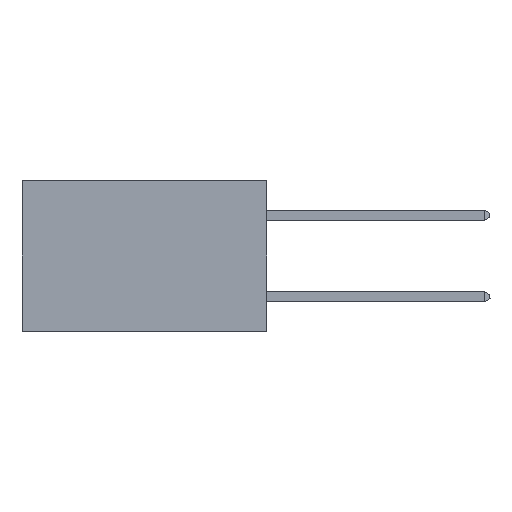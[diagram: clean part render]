
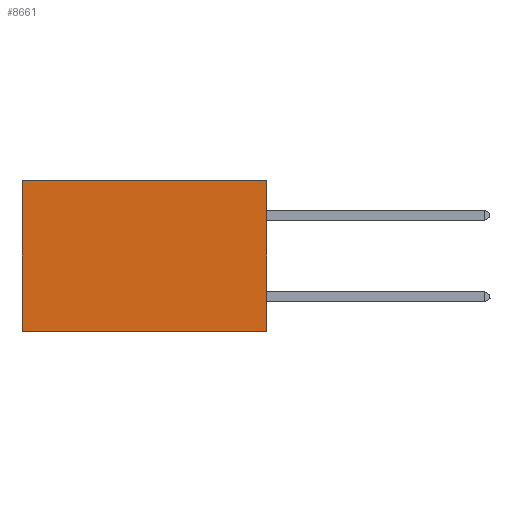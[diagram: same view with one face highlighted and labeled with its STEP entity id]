
A CAD part, left-side view. The second image highlights one B-rep face of the part: STEP entity #8661.
In plain terms, the highlighted planar face has unit normal (-1, 0, 0).
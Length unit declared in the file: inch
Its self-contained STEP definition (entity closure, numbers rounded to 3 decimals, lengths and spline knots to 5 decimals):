
#199 = CARTESIAN_POINT ( 'NONE',  ( 0.2875, 0., 0. ) ) ;
#417 = DIRECTION ( 'NONE',  ( 0., 0., -1. ) ) ;
#647 = VERTEX_POINT ( 'NONE', #5409 ) ;
#757 = EDGE_CURVE ( 'NONE', #14432, #23924, #18991, .T. ) ;
#1825 = LINE ( 'NONE', #18418, #25179 ) ;
#2025 = EDGE_CURVE ( 'NONE', #14432, #647, #1825, .T. ) ;
#2281 = VECTOR ( 'NONE', #417, 39.37008 ) ;
#3078 = VECTOR ( 'NONE', #3971, 39.37008 ) ;
#3748 = DIRECTION ( 'NONE',  ( 0., 0., -1. ) ) ;
#3971 = DIRECTION ( 'NONE',  ( 0., 1., 0. ) ) ;
#5409 = CARTESIAN_POINT ( 'NONE',  ( 0.2875, 0.6, 0. ) ) ;
#6171 = ORIENTED_EDGE ( 'NONE', *, *, #2025, .T. ) ;
#7472 = LINE ( 'NONE', #12927, #16571 ) ;
#7997 = FACE_OUTER_BOUND ( 'NONE', #15832, .T. ) ;
#8407 = PLANE ( 'NONE',  #21368 ) ;
#8661 = ADVANCED_FACE ( 'NONE', ( #7997 ), #8407, .F. ) ;
#9837 = EDGE_CURVE ( 'NONE', #23924, #15909, #25372, .T. ) ;
#9933 = ORIENTED_EDGE ( 'NONE', *, *, #757, .F. ) ;
#10668 = CARTESIAN_POINT ( 'NONE',  ( 0.2875, 0., 0. ) ) ;
#11431 = CARTESIAN_POINT ( 'NONE',  ( 0.2875, 0., 0. ) ) ;
#12497 = ORIENTED_EDGE ( 'NONE', *, *, #9837, .F. ) ;
#12574 = CARTESIAN_POINT ( 'NONE',  ( 0.2875, 0., -0.37 ) ) ;
#12927 = CARTESIAN_POINT ( 'NONE',  ( 0.2875, 0.6, 0. ) ) ;
#14432 = VERTEX_POINT ( 'NONE', #199 ) ;
#14695 = CARTESIAN_POINT ( 'NONE',  ( 0.2875, 0.6, -0.37 ) ) ;
#15832 = EDGE_LOOP ( 'NONE', ( #23559, #12497, #9933, #6171 ) ) ;
#15909 = VERTEX_POINT ( 'NONE', #14695 ) ;
#16571 = VECTOR ( 'NONE', #28467, 39.37008 ) ;
#16715 = EDGE_CURVE ( 'NONE', #647, #15909, #7472, .T. ) ;
#18418 = CARTESIAN_POINT ( 'NONE',  ( 0.2875, 0., 0. ) ) ;
#18991 = LINE ( 'NONE', #11431, #2281 ) ;
#21298 = CARTESIAN_POINT ( 'NONE',  ( 0.2875, 0., -0.37 ) ) ;
#21368 = AXIS2_PLACEMENT_3D ( 'NONE', #10668, #28075, #3748 ) ;
#23559 = ORIENTED_EDGE ( 'NONE', *, *, #16715, .T. ) ;
#23924 = VERTEX_POINT ( 'NONE', #21298 ) ;
#25118 = DIRECTION ( 'NONE',  ( 0., 1., 0. ) ) ;
#25179 = VECTOR ( 'NONE', #25118, 39.37008 ) ;
#25372 = LINE ( 'NONE', #12574, #3078 ) ;
#28075 = DIRECTION ( 'NONE',  ( 1., 0., 0. ) ) ;
#28467 = DIRECTION ( 'NONE',  ( 0., 0., -1. ) ) ;
